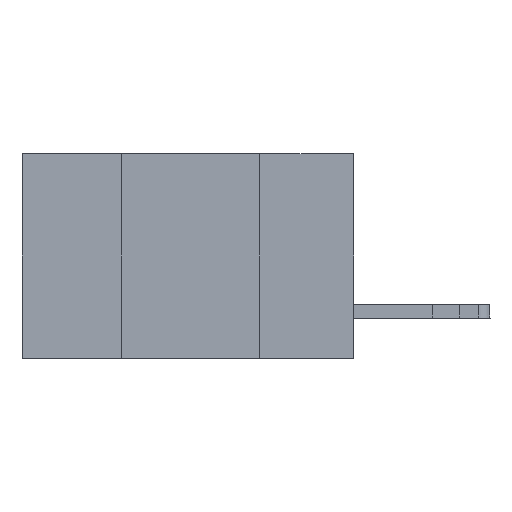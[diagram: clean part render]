
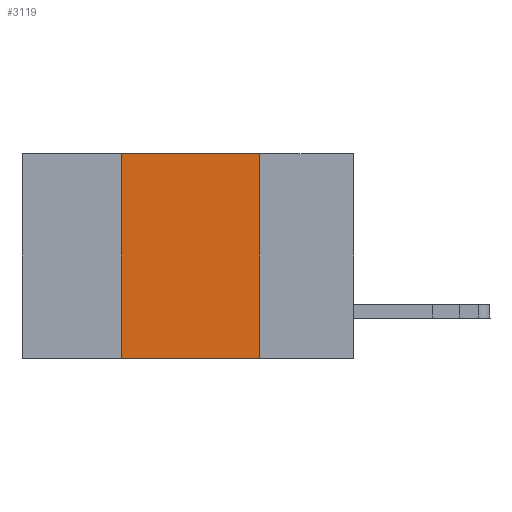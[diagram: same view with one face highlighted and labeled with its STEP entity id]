
A CAD part, left-side view. The second image highlights one B-rep face of the part: STEP entity #3119.
In plain terms, the highlighted planar face has unit normal (-1, 0, 0).
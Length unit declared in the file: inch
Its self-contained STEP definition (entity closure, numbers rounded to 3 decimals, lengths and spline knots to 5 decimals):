
#945 = EDGE_LOOP ( 'NONE', ( #8651, #9598, #4530, #3358 ) ) ;
#1368 = LINE ( 'NONE', #10459, #16445 ) ;
#2837 = DIRECTION ( 'NONE',  ( 0., -1., 0. ) ) ;
#3119 = ADVANCED_FACE ( 'NONE', ( #4185 ), #10675, .F. ) ;
#3352 = VECTOR ( 'NONE', #8839, 39.37008 ) ;
#3358 = ORIENTED_EDGE ( 'NONE', *, *, #5053, .T. ) ;
#4147 = VERTEX_POINT ( 'NONE', #12968 ) ;
#4185 = FACE_OUTER_BOUND ( 'NONE', #945, .T. ) ;
#4254 = VECTOR ( 'NONE', #16611, 39.37008 ) ;
#4369 = VERTEX_POINT ( 'NONE', #9769 ) ;
#4530 = ORIENTED_EDGE ( 'NONE', *, *, #12994, .F. ) ;
#4937 = DIRECTION ( 'NONE',  ( 0., -1., 0. ) ) ;
#5053 = EDGE_CURVE ( 'NONE', #4147, #4369, #1368, .T. ) ;
#6005 = VERTEX_POINT ( 'NONE', #7404 ) ;
#6858 = LINE ( 'NONE', #7960, #17046 ) ;
#7404 = CARTESIAN_POINT ( 'NONE',  ( 0., 0.17, 0. ) ) ;
#7960 = CARTESIAN_POINT ( 'NONE',  ( 0., 0.6, 0. ) ) ;
#8223 = DIRECTION ( 'NONE',  ( 1., 0., 0. ) ) ;
#8651 = ORIENTED_EDGE ( 'NONE', *, *, #18086, .F. ) ;
#8839 = DIRECTION ( 'NONE',  ( 0., 0., 1. ) ) ;
#9286 = CARTESIAN_POINT ( 'NONE',  ( 0., 0.42, 0. ) ) ;
#9598 = ORIENTED_EDGE ( 'NONE', *, *, #16533, .F. ) ;
#9769 = CARTESIAN_POINT ( 'NONE',  ( 0., 0.17, -0.37 ) ) ;
#10459 = CARTESIAN_POINT ( 'NONE',  ( 0., 0.6, -0.37 ) ) ;
#10675 = PLANE ( 'NONE',  #13982 ) ;
#10761 = VERTEX_POINT ( 'NONE', #9286 ) ;
#11243 = LINE ( 'NONE', #11649, #3352 ) ;
#11649 = CARTESIAN_POINT ( 'NONE',  ( 0., 0.42, 0. ) ) ;
#12199 = CARTESIAN_POINT ( 'NONE',  ( 0., 0.17, 0. ) ) ;
#12968 = CARTESIAN_POINT ( 'NONE',  ( 0., 0.42, -0.37 ) ) ;
#12994 = EDGE_CURVE ( 'NONE', #4147, #10761, #11243, .T. ) ;
#13982 = AXIS2_PLACEMENT_3D ( 'NONE', #17018, #8223, #14173 ) ;
#14173 = DIRECTION ( 'NONE',  ( 0., 0., -1. ) ) ;
#16076 = LINE ( 'NONE', #12199, #4254 ) ;
#16445 = VECTOR ( 'NONE', #2837, 39.37008 ) ;
#16533 = EDGE_CURVE ( 'NONE', #10761, #6005, #6858, .T. ) ;
#16611 = DIRECTION ( 'NONE',  ( 0., 0., -1. ) ) ;
#17018 = CARTESIAN_POINT ( 'NONE',  ( 0., 0.6, 0. ) ) ;
#17046 = VECTOR ( 'NONE', #4937, 39.37008 ) ;
#18086 = EDGE_CURVE ( 'NONE', #6005, #4369, #16076, .T. ) ;
